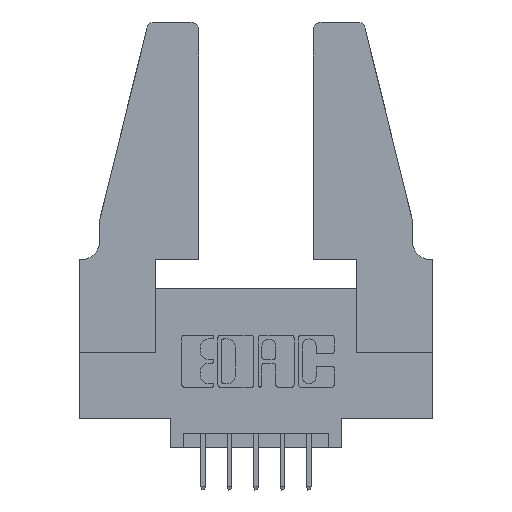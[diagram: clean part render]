
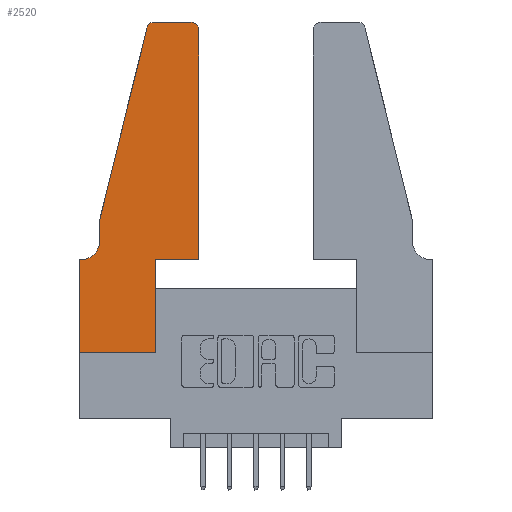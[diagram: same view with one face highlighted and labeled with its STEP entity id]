
A CAD part, top view. The second image highlights one B-rep face of the part: STEP entity #2520.
In plain terms, the highlighted planar face has unit normal (0, 0, 1).
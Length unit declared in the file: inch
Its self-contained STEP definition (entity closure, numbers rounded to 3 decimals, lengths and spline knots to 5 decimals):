
#16 = LINE ( 'NONE', #11259, #4094 ) ;
#37 = CARTESIAN_POINT ( 'NONE',  ( 0.4505, 0.35, 0.37 ) ) ;
#103 = VECTOR ( 'NONE', #6943, 39.37008 ) ;
#150 = CARTESIAN_POINT ( 'NONE',  ( 0., 0.35, 0.37 ) ) ;
#588 = EDGE_CURVE ( 'NONE', #1977, #1715, #2344, .T. ) ;
#606 = CIRCLE ( 'NONE', #8522, 0.07 ) ;
#744 = DIRECTION ( 'NONE',  ( -1., 0., 0. ) ) ;
#909 = DIRECTION ( 'NONE',  ( -1., 0., 0. ) ) ;
#1088 = ORIENTED_EDGE ( 'NONE', *, *, #10491, .T. ) ;
#1205 = DIRECTION ( 'NONE',  ( -1., 0., 0. ) ) ;
#1633 = DIRECTION ( 'NONE',  ( 0., 0., 1. ) ) ;
#1637 = DIRECTION ( 'NONE',  ( 0., 0., -1. ) ) ;
#1715 = VERTEX_POINT ( 'NONE', #2972 ) ;
#1788 = DIRECTION ( 'NONE',  ( 0., -1., 0. ) ) ;
#1881 = ORIENTED_EDGE ( 'NONE', *, *, #2241, .T. ) ;
#1893 = PLANE ( 'NONE',  #9626 ) ;
#1935 = CARTESIAN_POINT ( 'NONE',  ( 0.4505, 1.22, 0.37 ) ) ;
#1977 = VERTEX_POINT ( 'NONE', #9315 ) ;
#2003 = DIRECTION ( 'NONE',  ( 0., 0., 1. ) ) ;
#2241 = EDGE_CURVE ( 'NONE', #3958, #8741, #5825, .T. ) ;
#2344 = LINE ( 'NONE', #11167, #8890 ) ;
#2474 = CARTESIAN_POINT ( 'NONE',  ( 0.4505, 0.35, 0.37 ) ) ;
#2512 = CARTESIAN_POINT ( 'NONE',  ( 0., 0., 0.37 ) ) ;
#2520 = ADVANCED_FACE ( 'NONE', ( #2703 ), #1893, .T. ) ;
#2545 = ORIENTED_EDGE ( 'NONE', *, *, #6600, .T. ) ;
#2703 = FACE_OUTER_BOUND ( 'NONE', #7562, .T. ) ;
#2952 = VERTEX_POINT ( 'NONE', #7637 ) ;
#2972 = CARTESIAN_POINT ( 'NONE',  ( 0.284, 1.25, 0.37 ) ) ;
#3002 = AXIS2_PLACEMENT_3D ( 'NONE', #8662, #1633, #11117 ) ;
#3214 = CARTESIAN_POINT ( 'NONE',  ( 0.2865, 0., 0.37 ) ) ;
#3273 = DIRECTION ( 'NONE',  ( 1., 0., 0. ) ) ;
#3275 = VECTOR ( 'NONE', #11261, 39.37008 ) ;
#3350 = ORIENTED_EDGE ( 'NONE', *, *, #588, .T. ) ;
#3439 = CARTESIAN_POINT ( 'NONE',  ( 0.0755, 0.5, 0.37 ) ) ;
#3476 = CARTESIAN_POINT ( 'NONE',  ( 0.0055, 0.42, 0.37 ) ) ;
#3607 = VECTOR ( 'NONE', #6770, 39.37008 ) ;
#3901 = LINE ( 'NONE', #2474, #4432 ) ;
#3918 = VECTOR ( 'NONE', #5916, 39.37008 ) ;
#3958 = VERTEX_POINT ( 'NONE', #10084 ) ;
#4062 = LINE ( 'NONE', #10698, #7749 ) ;
#4094 = VECTOR ( 'NONE', #5652, 39.37008 ) ;
#4282 = CARTESIAN_POINT ( 'NONE',  ( 0.2865, 0.35, 0.37 ) ) ;
#4297 = CARTESIAN_POINT ( 'NONE',  ( 0.4205, 1.22, 0.37 ) ) ;
#4371 = VERTEX_POINT ( 'NONE', #37 ) ;
#4432 = VECTOR ( 'NONE', #10442, 39.37008 ) ;
#4724 = EDGE_CURVE ( 'NONE', #8741, #2952, #606, .T. ) ;
#4870 = CARTESIAN_POINT ( 'NONE',  ( 0., 0.35, 0.37 ) ) ;
#5004 = VERTEX_POINT ( 'NONE', #8188 ) ;
#5010 = ORIENTED_EDGE ( 'NONE', *, *, #7663, .T. ) ;
#5089 = ORIENTED_EDGE ( 'NONE', *, *, #10517, .T. ) ;
#5192 = EDGE_CURVE ( 'NONE', #5004, #3958, #9205, .T. ) ;
#5243 = EDGE_CURVE ( 'NONE', #10114, #1977, #8665, .T. ) ;
#5652 = DIRECTION ( 'NONE',  ( 0., 1., 0. ) ) ;
#5825 = LINE ( 'NONE', #7723, #7326 ) ;
#5916 = DIRECTION ( 'NONE',  ( 0., 1., 0. ) ) ;
#6176 = ORIENTED_EDGE ( 'NONE', *, *, #5192, .T. ) ;
#6600 = EDGE_CURVE ( 'NONE', #10371, #8985, #8428, .T. ) ;
#6630 = ORIENTED_EDGE ( 'NONE', *, *, #5243, .T. ) ;
#6770 = DIRECTION ( 'NONE',  ( -0.239, -0.971, 0. ) ) ;
#6834 = CARTESIAN_POINT ( 'NONE',  ( 0., 0., 0.37 ) ) ;
#6869 = CARTESIAN_POINT ( 'NONE',  ( 0., 0., 0.37 ) ) ;
#6943 = DIRECTION ( 'NONE',  ( 1., 0., 0. ) ) ;
#7326 = VECTOR ( 'NONE', #1788, 39.37008 ) ;
#7404 = AXIS2_PLACEMENT_3D ( 'NONE', #4297, #8499, #3273 ) ;
#7487 = EDGE_CURVE ( 'NONE', #10896, #10484, #8884, .T. ) ;
#7562 = EDGE_LOOP ( 'NONE', ( #3350, #8446, #6176, #1881, #9993, #7747, #8209, #5089, #2545, #1088, #5010, #6630 ) ) ;
#7637 = CARTESIAN_POINT ( 'NONE',  ( 0.0055, 0.35, 0.37 ) ) ;
#7663 = EDGE_CURVE ( 'NONE', #4371, #10114, #16, .T. ) ;
#7723 = CARTESIAN_POINT ( 'NONE',  ( 0.0755, 0.5, 0.37 ) ) ;
#7747 = ORIENTED_EDGE ( 'NONE', *, *, #8945, .T. ) ;
#7749 = VECTOR ( 'NONE', #1205, 39.37008 ) ;
#8020 = DIRECTION ( 'NONE',  ( 1., 0., 0. ) ) ;
#8188 = CARTESIAN_POINT ( 'NONE',  ( 0.25487, 1.22718, 0.37 ) ) ;
#8209 = ORIENTED_EDGE ( 'NONE', *, *, #7487, .T. ) ;
#8428 = LINE ( 'NONE', #4282, #3918 ) ;
#8446 = ORIENTED_EDGE ( 'NONE', *, *, #9169, .T. ) ;
#8499 = DIRECTION ( 'NONE',  ( 0., 0., 1. ) ) ;
#8522 = AXIS2_PLACEMENT_3D ( 'NONE', #3476, #1637, #909 ) ;
#8662 = CARTESIAN_POINT ( 'NONE',  ( 0.284, 1.22, 0.37 ) ) ;
#8665 = CIRCLE ( 'NONE', #7404, 0.03 ) ;
#8741 = VERTEX_POINT ( 'NONE', #10789 ) ;
#8884 = LINE ( 'NONE', #6834, #3275 ) ;
#8890 = VECTOR ( 'NONE', #744, 39.37008 ) ;
#8945 = EDGE_CURVE ( 'NONE', #2952, #10896, #4062, .T. ) ;
#8985 = VERTEX_POINT ( 'NONE', #9865 ) ;
#9169 = EDGE_CURVE ( 'NONE', #1715, #5004, #9384, .T. ) ;
#9205 = LINE ( 'NONE', #3439, #3607 ) ;
#9315 = CARTESIAN_POINT ( 'NONE',  ( 0.4205, 1.25, 0.37 ) ) ;
#9360 = LINE ( 'NONE', #6869, #103 ) ;
#9384 = CIRCLE ( 'NONE', #3002, 0.03 ) ;
#9626 = AXIS2_PLACEMENT_3D ( 'NONE', #150, #2003, #8020 ) ;
#9865 = CARTESIAN_POINT ( 'NONE',  ( 0.2865, 0.35, 0.37 ) ) ;
#9993 = ORIENTED_EDGE ( 'NONE', *, *, #4724, .T. ) ;
#10084 = CARTESIAN_POINT ( 'NONE',  ( 0.0755, 0.5, 0.37 ) ) ;
#10114 = VERTEX_POINT ( 'NONE', #1935 ) ;
#10371 = VERTEX_POINT ( 'NONE', #3214 ) ;
#10442 = DIRECTION ( 'NONE',  ( 1., 0., 0. ) ) ;
#10484 = VERTEX_POINT ( 'NONE', #2512 ) ;
#10491 = EDGE_CURVE ( 'NONE', #8985, #4371, #3901, .T. ) ;
#10517 = EDGE_CURVE ( 'NONE', #10484, #10371, #9360, .T. ) ;
#10698 = CARTESIAN_POINT ( 'NONE',  ( 0.0755, 0.35, 0.37 ) ) ;
#10789 = CARTESIAN_POINT ( 'NONE',  ( 0.0755, 0.42, 0.37 ) ) ;
#10896 = VERTEX_POINT ( 'NONE', #4870 ) ;
#11117 = DIRECTION ( 'NONE',  ( 1., 0., 0. ) ) ;
#11167 = CARTESIAN_POINT ( 'NONE',  ( 0.2605, 1.25, 0.37 ) ) ;
#11259 = CARTESIAN_POINT ( 'NONE',  ( 0.4505, 0.35, 0.37 ) ) ;
#11261 = DIRECTION ( 'NONE',  ( 0., -1., 0. ) ) ;
